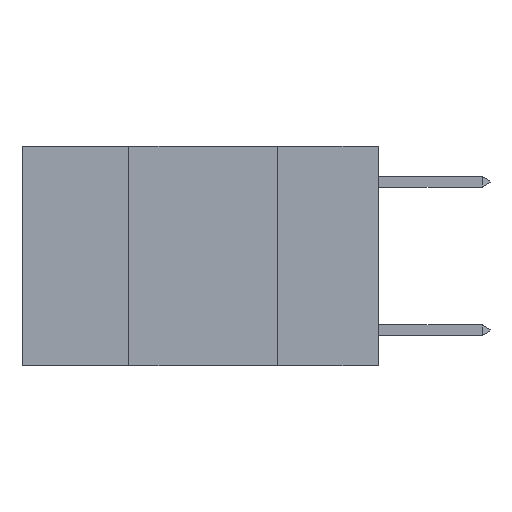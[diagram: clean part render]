
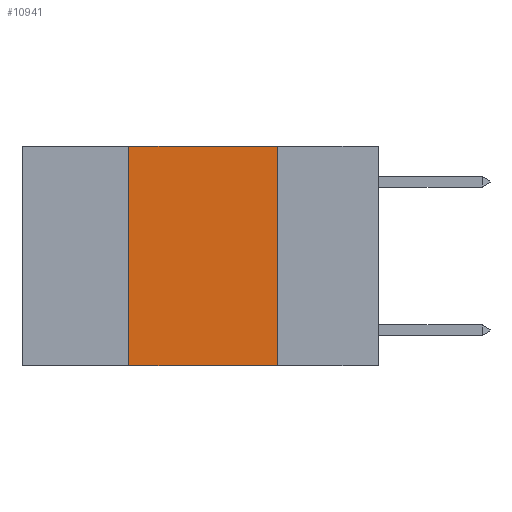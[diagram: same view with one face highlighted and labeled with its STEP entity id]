
A CAD part, left-side view. The second image highlights one B-rep face of the part: STEP entity #10941.
In plain terms, the highlighted planar face has unit normal (-1, 0, 0).
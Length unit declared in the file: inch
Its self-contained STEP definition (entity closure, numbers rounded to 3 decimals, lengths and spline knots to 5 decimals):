
#272 = CARTESIAN_POINT ( 'NONE',  ( 0., 0.42, -0.37 ) ) ;
#388 = CARTESIAN_POINT ( 'NONE',  ( 0., 0.42, 0. ) ) ;
#1014 = CARTESIAN_POINT ( 'NONE',  ( 0., 0.17, 0. ) ) ;
#2055 = FACE_OUTER_BOUND ( 'NONE', #8869, .T. ) ;
#2926 = DIRECTION ( 'NONE',  ( 0., 0., -1. ) ) ;
#4028 = VECTOR ( 'NONE', #20436, 39.37008 ) ;
#6765 = LINE ( 'NONE', #10526, #18574 ) ;
#7038 = VERTEX_POINT ( 'NONE', #388 ) ;
#7140 = CARTESIAN_POINT ( 'NONE',  ( 0., 0.6, -0.37 ) ) ;
#8869 = EDGE_LOOP ( 'NONE', ( #26849, #27073, #27436, #27622 ) ) ;
#9690 = CARTESIAN_POINT ( 'NONE',  ( 0., 0.6, 0. ) ) ;
#10526 = CARTESIAN_POINT ( 'NONE',  ( 0., 0.6, 0. ) ) ;
#10941 = ADVANCED_FACE ( 'NONE', ( #2055 ), #14138, .F. ) ;
#11125 = EDGE_CURVE ( 'NONE', #27673, #7038, #21640, .T. ) ;
#13061 = CARTESIAN_POINT ( 'NONE',  ( 0., 0.17, 0. ) ) ;
#14138 = PLANE ( 'NONE',  #23059 ) ;
#15043 = VECTOR ( 'NONE', #21364, 39.37008 ) ;
#15233 = DIRECTION ( 'NONE',  ( 0., 0., -1. ) ) ;
#15245 = LINE ( 'NONE', #7140, #4028 ) ;
#15519 = EDGE_CURVE ( 'NONE', #27673, #18096, #15245, .T. ) ;
#16323 = DIRECTION ( 'NONE',  ( 1., 0., 0. ) ) ;
#18096 = VERTEX_POINT ( 'NONE', #19072 ) ;
#18574 = VECTOR ( 'NONE', #25995, 39.37008 ) ;
#19072 = CARTESIAN_POINT ( 'NONE',  ( 0., 0.17, -0.37 ) ) ;
#20436 = DIRECTION ( 'NONE',  ( 0., -1., 0. ) ) ;
#21255 = VERTEX_POINT ( 'NONE', #1014 ) ;
#21364 = DIRECTION ( 'NONE',  ( 0., 0., 1. ) ) ;
#21640 = LINE ( 'NONE', #25738, #15043 ) ;
#22626 = LINE ( 'NONE', #13061, #27798 ) ;
#23059 = AXIS2_PLACEMENT_3D ( 'NONE', #9690, #16323, #2926 ) ;
#24468 = EDGE_CURVE ( 'NONE', #21255, #18096, #22626, .T. ) ;
#25738 = CARTESIAN_POINT ( 'NONE',  ( 0., 0.42, 0. ) ) ;
#25995 = DIRECTION ( 'NONE',  ( 0., -1., 0. ) ) ;
#26849 = ORIENTED_EDGE ( 'NONE', *, *, #24468, .F. ) ;
#27073 = ORIENTED_EDGE ( 'NONE', *, *, #27998, .F. ) ;
#27436 = ORIENTED_EDGE ( 'NONE', *, *, #11125, .F. ) ;
#27622 = ORIENTED_EDGE ( 'NONE', *, *, #15519, .T. ) ;
#27673 = VERTEX_POINT ( 'NONE', #272 ) ;
#27798 = VECTOR ( 'NONE', #15233, 39.37008 ) ;
#27998 = EDGE_CURVE ( 'NONE', #7038, #21255, #6765, .T. ) ;
